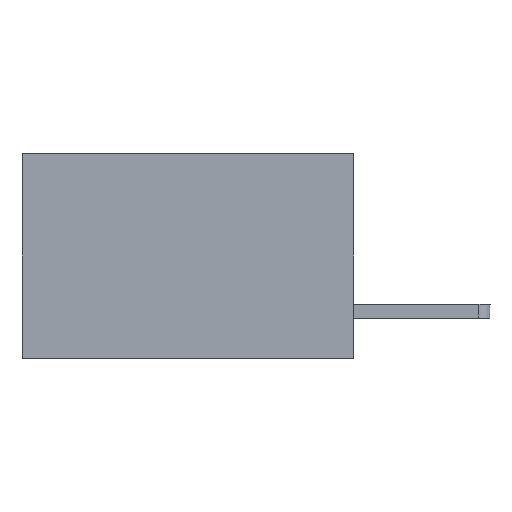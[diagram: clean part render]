
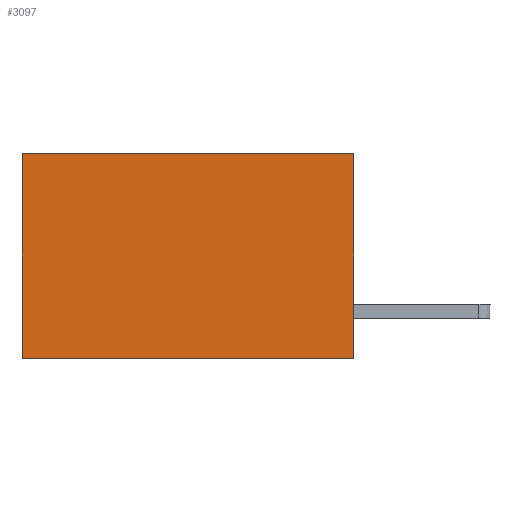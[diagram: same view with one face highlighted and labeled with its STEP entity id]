
A CAD part, left-side view. The second image highlights one B-rep face of the part: STEP entity #3097.
In plain terms, the highlighted planar face has unit normal (-1, 0, 0).
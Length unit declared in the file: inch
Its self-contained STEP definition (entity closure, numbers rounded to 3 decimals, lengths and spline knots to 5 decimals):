
#219 = VERTEX_POINT ( 'NONE', #6138 ) ;
#409 = LINE ( 'NONE', #856, #9981 ) ;
#473 = CARTESIAN_POINT ( 'NONE',  ( 0.2875, 0.6, 0. ) ) ;
#615 = ORIENTED_EDGE ( 'NONE', *, *, #3520, .F. ) ;
#856 = CARTESIAN_POINT ( 'NONE',  ( 0.2875, 0., 0. ) ) ;
#1116 = ORIENTED_EDGE ( 'NONE', *, *, #5866, .F. ) ;
#1200 = LINE ( 'NONE', #9143, #1993 ) ;
#1341 = LINE ( 'NONE', #473, #3958 ) ;
#1709 = DIRECTION ( 'NONE',  ( 1., 0., 0. ) ) ;
#1993 = VECTOR ( 'NONE', #3452, 39.37008 ) ;
#2274 = DIRECTION ( 'NONE',  ( 0., 1., 0. ) ) ;
#2772 = EDGE_LOOP ( 'NONE', ( #3105, #1116, #615, #9283 ) ) ;
#2981 = AXIS2_PLACEMENT_3D ( 'NONE', #6719, #1709, #4088 ) ;
#3095 = EDGE_CURVE ( 'NONE', #7295, #8099, #1341, .T. ) ;
#3097 = ADVANCED_FACE ( 'NONE', ( #7893 ), #5832, .F. ) ;
#3105 = ORIENTED_EDGE ( 'NONE', *, *, #3095, .T. ) ;
#3452 = DIRECTION ( 'NONE',  ( 0., 1., 0. ) ) ;
#3520 = EDGE_CURVE ( 'NONE', #5641, #219, #409, .T. ) ;
#3891 = CARTESIAN_POINT ( 'NONE',  ( 0.2875, 0.6, -0.37 ) ) ;
#3958 = VECTOR ( 'NONE', #8896, 39.37008 ) ;
#4088 = DIRECTION ( 'NONE',  ( 0., 0., -1. ) ) ;
#4145 = DIRECTION ( 'NONE',  ( 0., 0., -1. ) ) ;
#5641 = VERTEX_POINT ( 'NONE', #5807 ) ;
#5807 = CARTESIAN_POINT ( 'NONE',  ( 0.2875, 0., 0. ) ) ;
#5832 = PLANE ( 'NONE',  #2981 ) ;
#5866 = EDGE_CURVE ( 'NONE', #219, #8099, #6519, .T. ) ;
#6138 = CARTESIAN_POINT ( 'NONE',  ( 0.2875, 0., -0.37 ) ) ;
#6519 = LINE ( 'NONE', #10673, #8765 ) ;
#6719 = CARTESIAN_POINT ( 'NONE',  ( 0.2875, 0., 0. ) ) ;
#7295 = VERTEX_POINT ( 'NONE', #10185 ) ;
#7893 = FACE_OUTER_BOUND ( 'NONE', #2772, .T. ) ;
#8099 = VERTEX_POINT ( 'NONE', #3891 ) ;
#8267 = EDGE_CURVE ( 'NONE', #5641, #7295, #1200, .T. ) ;
#8765 = VECTOR ( 'NONE', #2274, 39.37008 ) ;
#8896 = DIRECTION ( 'NONE',  ( 0., 0., -1. ) ) ;
#9143 = CARTESIAN_POINT ( 'NONE',  ( 0.2875, 0., 0. ) ) ;
#9283 = ORIENTED_EDGE ( 'NONE', *, *, #8267, .T. ) ;
#9981 = VECTOR ( 'NONE', #4145, 39.37008 ) ;
#10185 = CARTESIAN_POINT ( 'NONE',  ( 0.2875, 0.6, 0. ) ) ;
#10673 = CARTESIAN_POINT ( 'NONE',  ( 0.2875, 0., -0.37 ) ) ;
